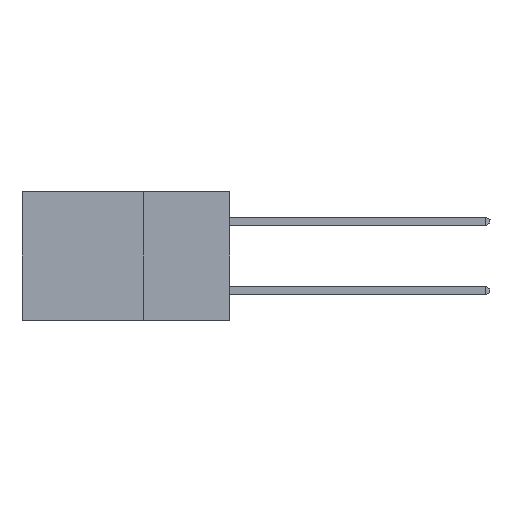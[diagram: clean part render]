
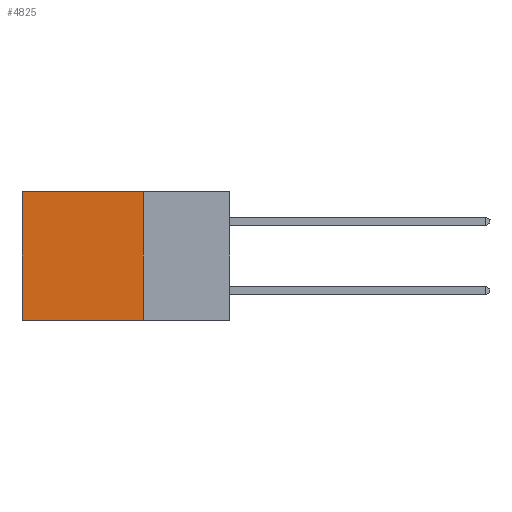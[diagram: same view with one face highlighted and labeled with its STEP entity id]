
A CAD part, left-side view. The second image highlights one B-rep face of the part: STEP entity #4825.
In plain terms, the highlighted planar face has unit normal (-1, 0, 0).
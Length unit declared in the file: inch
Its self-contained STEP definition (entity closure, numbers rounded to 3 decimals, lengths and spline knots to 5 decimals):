
#174 = ORIENTED_EDGE ( 'NONE', *, *, #8526, .F. ) ;
#224 = DIRECTION ( 'NONE',  ( 0., 0., -1. ) ) ;
#331 = CARTESIAN_POINT ( 'NONE',  ( 0.298, 0.6, 0. ) ) ;
#757 = DIRECTION ( 'NONE',  ( 0., 0., -1. ) ) ;
#1998 = CARTESIAN_POINT ( 'NONE',  ( 0.298, 0.6, -0.37 ) ) ;
#2077 = LINE ( 'NONE', #3990, #4230 ) ;
#2361 = ORIENTED_EDGE ( 'NONE', *, *, #10556, .T. ) ;
#2649 = VERTEX_POINT ( 'NONE', #10158 ) ;
#2964 = LINE ( 'NONE', #12755, #9269 ) ;
#3520 = CARTESIAN_POINT ( 'NONE',  ( 0.298, 0.25, 0. ) ) ;
#3566 = AXIS2_PLACEMENT_3D ( 'NONE', #7573, #9705, #224 ) ;
#3990 = CARTESIAN_POINT ( 'NONE',  ( 0.298, 0.6, 0. ) ) ;
#4230 = VECTOR ( 'NONE', #757, 39.37008 ) ;
#4825 = ADVANCED_FACE ( 'NONE', ( #13287 ), #6518, .F. ) ;
#5061 = DIRECTION ( 'NONE',  ( 0., 1., 0. ) ) ;
#5559 = VERTEX_POINT ( 'NONE', #3520 ) ;
#6518 = PLANE ( 'NONE',  #3566 ) ;
#6541 = VERTEX_POINT ( 'NONE', #1998 ) ;
#6807 = VERTEX_POINT ( 'NONE', #331 ) ;
#6861 = LINE ( 'NONE', #13416, #11043 ) ;
#7573 = CARTESIAN_POINT ( 'NONE',  ( 0.298, 0.25, 0. ) ) ;
#7713 = EDGE_CURVE ( 'NONE', #6807, #6541, #2077, .T. ) ;
#8526 = EDGE_CURVE ( 'NONE', #5559, #2649, #6861, .T. ) ;
#9187 = EDGE_CURVE ( 'NONE', #2649, #6541, #12008, .T. ) ;
#9191 = DIRECTION ( 'NONE',  ( 0., 0., -1. ) ) ;
#9206 = EDGE_LOOP ( 'NONE', ( #10753, #12886, #174, #2361 ) ) ;
#9254 = CARTESIAN_POINT ( 'NONE',  ( 0.298, 0.25, -0.37 ) ) ;
#9269 = VECTOR ( 'NONE', #9550, 39.37008 ) ;
#9550 = DIRECTION ( 'NONE',  ( 0., 1., 0. ) ) ;
#9705 = DIRECTION ( 'NONE',  ( 1., 0., 0. ) ) ;
#10158 = CARTESIAN_POINT ( 'NONE',  ( 0.298, 0.25, -0.37 ) ) ;
#10556 = EDGE_CURVE ( 'NONE', #5559, #6807, #2964, .T. ) ;
#10753 = ORIENTED_EDGE ( 'NONE', *, *, #7713, .T. ) ;
#11043 = VECTOR ( 'NONE', #9191, 39.37008 ) ;
#12008 = LINE ( 'NONE', #9254, #12517 ) ;
#12517 = VECTOR ( 'NONE', #5061, 39.37008 ) ;
#12755 = CARTESIAN_POINT ( 'NONE',  ( 0.298, 0.25, 0. ) ) ;
#12886 = ORIENTED_EDGE ( 'NONE', *, *, #9187, .F. ) ;
#13287 = FACE_OUTER_BOUND ( 'NONE', #9206, .T. ) ;
#13416 = CARTESIAN_POINT ( 'NONE',  ( 0.298, 0.25, 0. ) ) ;
